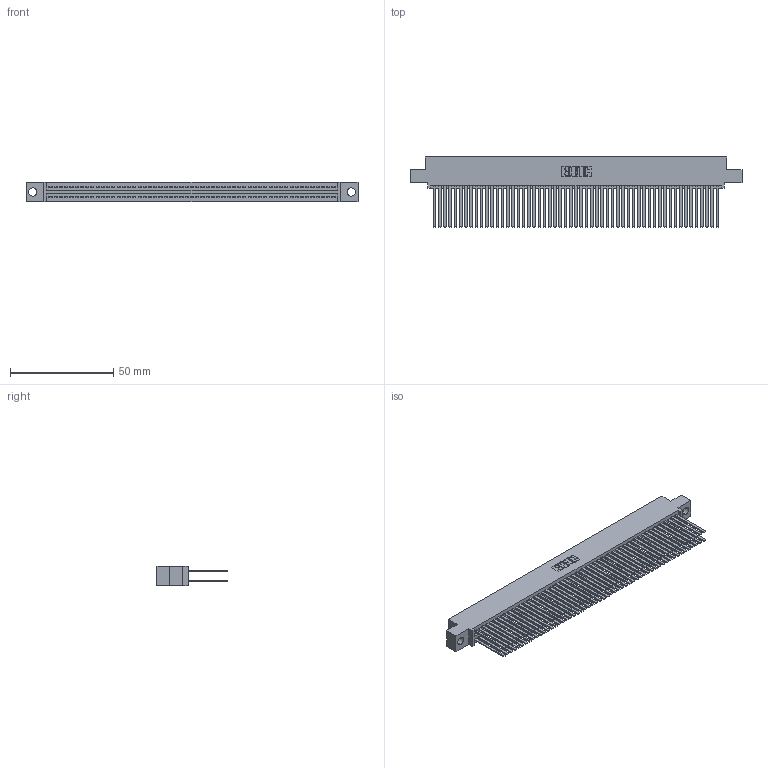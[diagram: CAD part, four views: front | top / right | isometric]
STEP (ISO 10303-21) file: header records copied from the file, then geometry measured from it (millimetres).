
FILE_DESCRIPTION (( 'STEP AP203' ), '1' );
FILE_NAME ('345-110-544-504.STEP', '2021-05-21T15:15:21', ( '' ), ( '' ), 'SwSTEP 2.0', 'SolidWorks 2020', '' );
FILE_SCHEMA (( 'CONFIG_CONTROL_DESIGN' ));
Length unit declared in the file: inch
Products named in the file (3): 345 Part_0.110 Offset - 0.156 Dia-TI; 345-292-001_345-293-144; 345-110-544-504
Assembly tree (111 placements, depth 2):
  345-110-544-504
    345 Part_0.110 Offset - 0.156 Dia-TI
    345-292-001_345-293-144  x110
Bounding box: 160.91 x 33.96 x 9.4 mm (x, y, z)
Volume: 17114.2 mm3; surface area: 30013.4 mm2
Topology: 111 solids, 111 shells, 4984 faces, 14799 edges, 9718 vertices
Faces by surface type: plane 3288, cylinder 1696
Entity records: 41771 total; most frequent: CARTESIAN_POINT 6994, ORIENTED_EDGE 6926, DIRECTION 6147, EDGE_CURVE 3463, LINE 3115, VECTOR 3115, VERTEX_POINT 2306, AXIS2_PLACEMENT_3D 1516
